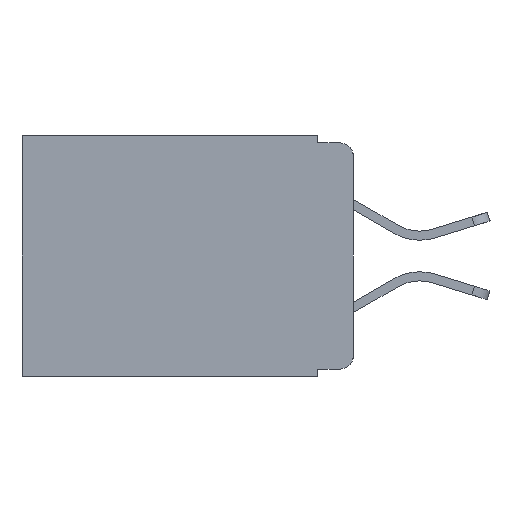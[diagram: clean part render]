
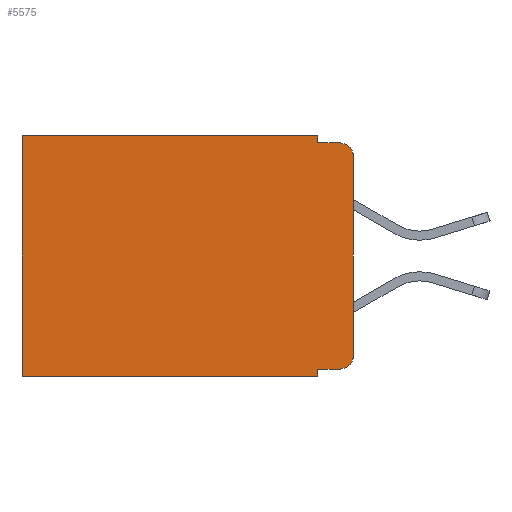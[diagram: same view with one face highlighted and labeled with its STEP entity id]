
A CAD part, left-side view. The second image highlights one B-rep face of the part: STEP entity #5575.
In plain terms, the highlighted planar face has unit normal (-1, 0, 0).
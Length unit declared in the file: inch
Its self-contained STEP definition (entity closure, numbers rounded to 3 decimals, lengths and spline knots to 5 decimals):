
#7 = DIRECTION ( 'NONE',  ( 0., -1., 0. ) ) ;
#151 = CARTESIAN_POINT ( 'NONE',  ( 0.298, 0., -0.313 ) ) ;
#224 = CARTESIAN_POINT ( 'NONE',  ( 0.298, 0., 0. ) ) ;
#718 = VERTEX_POINT ( 'NONE', #8403 ) ;
#809 = CARTESIAN_POINT ( 'NONE',  ( 0.298, 0.051, -0.343 ) ) ;
#872 = CARTESIAN_POINT ( 'NONE',  ( 0.298, 0., -0.343 ) ) ;
#938 = VECTOR ( 'NONE', #7, 39.37008 ) ;
#1278 = CARTESIAN_POINT ( 'NONE',  ( 0.298, 0.051, -0.01 ) ) ;
#1476 = EDGE_CURVE ( 'NONE', #718, #2244, #3253, .T. ) ;
#1589 = EDGE_CURVE ( 'NONE', #5874, #9940, #8758, .T. ) ;
#1666 = EDGE_CURVE ( 'NONE', #718, #5874, #10323, .T. ) ;
#1669 = VERTEX_POINT ( 'NONE', #6156 ) ;
#1828 = LINE ( 'NONE', #224, #9757 ) ;
#1833 = CARTESIAN_POINT ( 'NONE',  ( 0.298, 0.473, 0. ) ) ;
#1950 = EDGE_LOOP ( 'NONE', ( #9588, #3735, #6629, #3391, #4584, #8524, #7387, #7370, #10437, #3824 ) ) ;
#1951 = EDGE_CURVE ( 'NONE', #9355, #4198, #5754, .T. ) ;
#2099 = CARTESIAN_POINT ( 'NONE',  ( 0.298, 0.051, -0.333 ) ) ;
#2244 = VERTEX_POINT ( 'NONE', #2981 ) ;
#2301 = CIRCLE ( 'NONE', #3704, 0.02 ) ;
#2312 = CARTESIAN_POINT ( 'NONE',  ( 0.298, 0.051, -0.01 ) ) ;
#2588 = DIRECTION ( 'NONE',  ( -1., 0., 0. ) ) ;
#2871 = CARTESIAN_POINT ( 'NONE',  ( 0.298, 0.473, 0. ) ) ;
#2910 = LINE ( 'NONE', #8300, #8922 ) ;
#2940 = LINE ( 'NONE', #1833, #4945 ) ;
#2981 = CARTESIAN_POINT ( 'NONE',  ( 0.298, 0.02, -0.333 ) ) ;
#3253 = LINE ( 'NONE', #2099, #938 ) ;
#3264 = AXIS2_PLACEMENT_3D ( 'NONE', #9689, #4920, #10464 ) ;
#3358 = PLANE ( 'NONE',  #6455 ) ;
#3391 = ORIENTED_EDGE ( 'NONE', *, *, #5918, .F. ) ;
#3599 = DIRECTION ( 'NONE',  ( 0., 0., -1. ) ) ;
#3704 = AXIS2_PLACEMENT_3D ( 'NONE', #7526, #2588, #8345 ) ;
#3735 = ORIENTED_EDGE ( 'NONE', *, *, #7927, .T. ) ;
#3824 = ORIENTED_EDGE ( 'NONE', *, *, #8355, .T. ) ;
#4048 = CIRCLE ( 'NONE', #3264, 0.02 ) ;
#4104 = DIRECTION ( 'NONE',  ( 0., -1., 0. ) ) ;
#4198 = VERTEX_POINT ( 'NONE', #2871 ) ;
#4325 = DIRECTION ( 'NONE',  ( 0., 1., 0. ) ) ;
#4532 = VERTEX_POINT ( 'NONE', #1278 ) ;
#4584 = ORIENTED_EDGE ( 'NONE', *, *, #1951, .T. ) ;
#4920 = DIRECTION ( 'NONE',  ( -1., 0., 0. ) ) ;
#4945 = VECTOR ( 'NONE', #3599, 39.37008 ) ;
#5028 = EDGE_CURVE ( 'NONE', #4532, #1669, #6922, .T. ) ;
#5461 = DIRECTION ( 'NONE',  ( 0., 0., -1. ) ) ;
#5575 = ADVANCED_FACE ( 'NONE', ( #10256 ), #3358, .F. ) ;
#5754 = LINE ( 'NONE', #10131, #8135 ) ;
#5874 = VERTEX_POINT ( 'NONE', #809 ) ;
#5918 = EDGE_CURVE ( 'NONE', #9355, #4532, #2910, .T. ) ;
#6139 = VECTOR ( 'NONE', #10225, 39.37008 ) ;
#6156 = CARTESIAN_POINT ( 'NONE',  ( 0.298, 0.02, -0.01 ) ) ;
#6219 = CARTESIAN_POINT ( 'NONE',  ( 0.298, 0.473, -0.343 ) ) ;
#6455 = AXIS2_PLACEMENT_3D ( 'NONE', #8774, #9493, #9470 ) ;
#6542 = VERTEX_POINT ( 'NONE', #8089 ) ;
#6629 = ORIENTED_EDGE ( 'NONE', *, *, #5028, .F. ) ;
#6634 = VECTOR ( 'NONE', #4325, 39.37008 ) ;
#6686 = VECTOR ( 'NONE', #4104, 39.37008 ) ;
#6922 = LINE ( 'NONE', #2312, #6686 ) ;
#6974 = CARTESIAN_POINT ( 'NONE',  ( 0.298, 0.051, 0. ) ) ;
#7370 = ORIENTED_EDGE ( 'NONE', *, *, #1666, .F. ) ;
#7387 = ORIENTED_EDGE ( 'NONE', *, *, #1589, .F. ) ;
#7448 = DIRECTION ( 'NONE',  ( 0., 1., 0. ) ) ;
#7526 = CARTESIAN_POINT ( 'NONE',  ( 0.298, 0.02, -0.03 ) ) ;
#7881 = DIRECTION ( 'NONE',  ( 0., 0., -1. ) ) ;
#7927 = EDGE_CURVE ( 'NONE', #6542, #1669, #2301, .T. ) ;
#8089 = CARTESIAN_POINT ( 'NONE',  ( 0.298, 0., -0.03 ) ) ;
#8135 = VECTOR ( 'NONE', #7448, 39.37008 ) ;
#8300 = CARTESIAN_POINT ( 'NONE',  ( 0.298, 0.051, 0. ) ) ;
#8345 = DIRECTION ( 'NONE',  ( 0., 0., -1. ) ) ;
#8355 = EDGE_CURVE ( 'NONE', #2244, #10500, #4048, .T. ) ;
#8403 = CARTESIAN_POINT ( 'NONE',  ( 0.298, 0.051, -0.333 ) ) ;
#8524 = ORIENTED_EDGE ( 'NONE', *, *, #9254, .T. ) ;
#8758 = LINE ( 'NONE', #872, #6634 ) ;
#8774 = CARTESIAN_POINT ( 'NONE',  ( 0.298, 0., 0. ) ) ;
#8922 = VECTOR ( 'NONE', #7881, 39.37008 ) ;
#9254 = EDGE_CURVE ( 'NONE', #4198, #9940, #2940, .T. ) ;
#9355 = VERTEX_POINT ( 'NONE', #10123 ) ;
#9470 = DIRECTION ( 'NONE',  ( 0., 0., -1. ) ) ;
#9493 = DIRECTION ( 'NONE',  ( 1., 0., 0. ) ) ;
#9588 = ORIENTED_EDGE ( 'NONE', *, *, #10561, .F. ) ;
#9689 = CARTESIAN_POINT ( 'NONE',  ( 0.298, 0.02, -0.313 ) ) ;
#9757 = VECTOR ( 'NONE', #5461, 39.37008 ) ;
#9940 = VERTEX_POINT ( 'NONE', #6219 ) ;
#10123 = CARTESIAN_POINT ( 'NONE',  ( 0.298, 0.051, 0. ) ) ;
#10131 = CARTESIAN_POINT ( 'NONE',  ( 0.298, 0., 0. ) ) ;
#10225 = DIRECTION ( 'NONE',  ( 0., 0., -1. ) ) ;
#10256 = FACE_OUTER_BOUND ( 'NONE', #1950, .T. ) ;
#10323 = LINE ( 'NONE', #6974, #6139 ) ;
#10437 = ORIENTED_EDGE ( 'NONE', *, *, #1476, .T. ) ;
#10464 = DIRECTION ( 'NONE',  ( 0., 0., -1. ) ) ;
#10500 = VERTEX_POINT ( 'NONE', #151 ) ;
#10561 = EDGE_CURVE ( 'NONE', #6542, #10500, #1828, .T. ) ;
